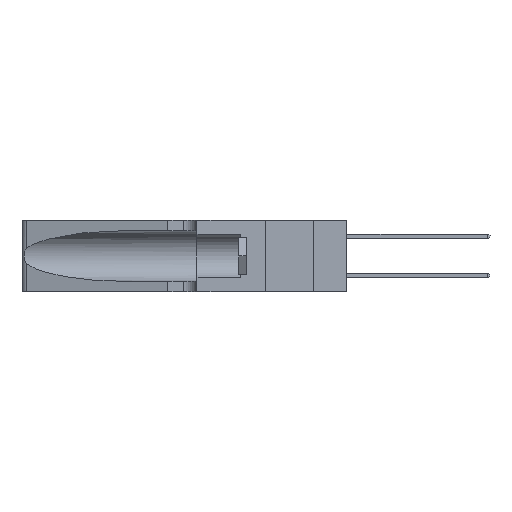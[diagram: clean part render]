
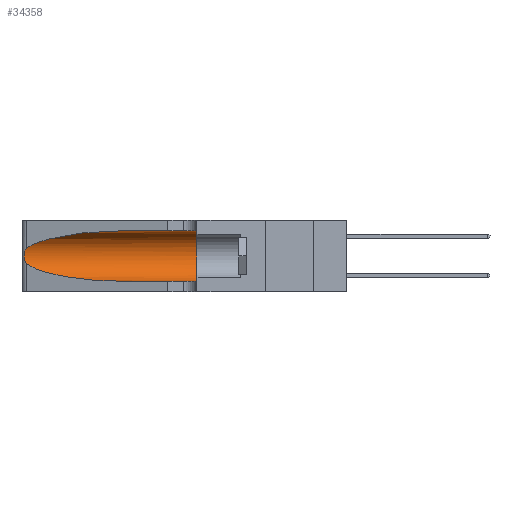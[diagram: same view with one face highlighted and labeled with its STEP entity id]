
A CAD part, left-side view. The second image highlights one B-rep face of the part: STEP entity #34358.
In plain terms, the highlighted cylindrical face has radius 3.308 mm (diameter 6.617 mm), a partial arc.
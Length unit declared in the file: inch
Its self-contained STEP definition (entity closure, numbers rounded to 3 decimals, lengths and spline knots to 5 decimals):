
#531 = ORIENTED_EDGE ( 'NONE', *, *, #25569, .T. ) ;
#635 = DIRECTION ( 'NONE',  ( 0., -1., 0. ) ) ;
#1025 = EDGE_CURVE ( 'NONE', #2782, #19241, #13619, .T. ) ;
#1356 = CARTESIAN_POINT ( 'NONE',  ( 0.1305, 0.35, 0.31525 ) ) ;
#1632 = CARTESIAN_POINT ( 'NONE',  ( 0.1305, 0.72297, 0.05475 ) ) ;
#2381 = CARTESIAN_POINT ( 'NONE',  ( 0.25487, 1.22718, 0.14631 ) ) ;
#2574 = AXIS2_PLACEMENT_3D ( 'NONE', #5266, #4666, #28445 ) ;
#2782 = VERTEX_POINT ( 'NONE', #18855 ) ;
#3569 = VERTEX_POINT ( 'NONE', #1356 ) ;
#4320 = CARTESIAN_POINT ( 'NONE',  ( 0.2373, 1.15595, 0.28018 ) ) ;
#4666 = DIRECTION ( 'NONE',  ( 0., 1., 0. ) ) ;
#5266 = CARTESIAN_POINT ( 'NONE',  ( 0.1305, 0.35, 0.185 ) ) ;
#6025 = CARTESIAN_POINT ( 'NONE',  ( 0.26017, 1.23833, 0.17102 ) ) ;
#6101 = ORIENTED_EDGE ( 'NONE', *, *, #24905, .T. ) ;
#6287 = ORIENTED_EDGE ( 'NONE', *, *, #32397, .F. ) ;
#6356 = VERTEX_POINT ( 'NONE', #2381 ) ;
#6449 = CARTESIAN_POINT ( 'NONE',  ( 0.25639, 1.23186, 0.15144 ) ) ;
#8166 = CARTESIAN_POINT ( 'NONE',  ( 0.1305, 0.72297, 0.31525 ) ) ;
#9564 = CARTESIAN_POINT ( 'NONE',  ( 0.25856, 1.23593, 0.16098 ) ) ;
#9710 = CARTESIAN_POINT ( 'NONE',  ( 0.26075, 1.23896, 0.19203 ) ) ;
#11572 = CIRCLE ( 'NONE', #2574, 0.13025 ) ;
#12042 = CARTESIAN_POINT ( 'NONE',  ( 0.25487, 1.22718, 0.14631 ) ) ;
#13156 = VERTEX_POINT ( 'NONE', #18201 ) ;
#13256 = CARTESIAN_POINT ( 'NONE',  ( 0.25487, 1.22718, 0.14631 ) ) ;
#13619 =( BOUNDED_CURVE ( )  B_SPLINE_CURVE ( 3, ( #8166, #24989, #4320, #18243 ),
 .UNSPECIFIED., .F., .F. ) 
 B_SPLINE_CURVE_WITH_KNOTS ( ( 4, 4 ),
 ( 1.5708, 2.84003 ),
 .UNSPECIFIED. ) 
 CURVE ( )  GEOMETRIC_REPRESENTATION_ITEM ( )  RATIONAL_B_SPLINE_CURVE ( ( 1., 0.87, 0.87, 1. ) ) 
 REPRESENTATION_ITEM ( '' )  );
#13638 = VECTOR ( 'NONE', #31619, 39.37008 ) ;
#15139 = CARTESIAN_POINT ( 'NONE',  ( 0.25639, 1.23184, 0.21858 ) ) ;
#15176 = CYLINDRICAL_SURFACE ( 'NONE', #16251, 0.13025 ) ;
#15279 = CARTESIAN_POINT ( 'NONE',  ( 0.25787, 1.23484, 0.2124 ) ) ;
#15413 = EDGE_CURVE ( 'NONE', #2782, #3569, #27504, .T. ) ;
#15910 = DIRECTION ( 'NONE',  ( 0., 0., -1. ) ) ;
#16251 = AXIS2_PLACEMENT_3D ( 'NONE', #25642, #19061, #15910 ) ;
#18201 = CARTESIAN_POINT ( 'NONE',  ( 0.1305, 0.35, 0.05475 ) ) ;
#18243 = CARTESIAN_POINT ( 'NONE',  ( 0.25487, 1.22718, 0.22369 ) ) ;
#18705 = CARTESIAN_POINT ( 'NONE',  ( 0.25854, 1.2359, 0.20912 ) ) ;
#18855 = CARTESIAN_POINT ( 'NONE',  ( 0.1305, 0.72297, 0.31525 ) ) ;
#19061 = DIRECTION ( 'NONE',  ( 0., -1., 0. ) ) ;
#19241 = VERTEX_POINT ( 'NONE', #28084 ) ;
#20495 = FACE_OUTER_BOUND ( 'NONE', #32352, .T. ) ;
#22337 = CARTESIAN_POINT ( 'NONE',  ( 0.2373, 1.15595, 0.08982 ) ) ;
#24264 = B_SPLINE_CURVE_WITH_KNOTS ( 'NONE', 3,
 ( #28708, #35617, #15139, #15279, #18705, #30000, #9710, #26829, #6025, #9564, #40023, #6449, #33584, #13256 ),
 .UNSPECIFIED., .F., .F.,
 ( 4, 2, 2, 2, 2, 2, 4 ),
 ( 0., 0.00027, 0.00053, 0.00107, 0.0016, 0.00187, 0.00214 ),
 .UNSPECIFIED. ) ;
#24905 = EDGE_CURVE ( 'NONE', #19241, #6356, #24264, .T. ) ;
#24989 = CARTESIAN_POINT ( 'NONE',  ( 0.18966, 0.96281, 0.31525 ) ) ;
#25569 = EDGE_CURVE ( 'NONE', #6356, #31322, #42159, .T. ) ;
#25642 = CARTESIAN_POINT ( 'NONE',  ( 0.1305, 1.61858, 0.185 ) ) ;
#26042 = EDGE_CURVE ( 'NONE', #31322, #13156, #37537, .T. ) ;
#26687 = ORIENTED_EDGE ( 'NONE', *, *, #15413, .F. ) ;
#26829 = CARTESIAN_POINT ( 'NONE',  ( 0.26075, 1.23896, 0.178 ) ) ;
#27504 = LINE ( 'NONE', #41184, #13638 ) ;
#27622 = ORIENTED_EDGE ( 'NONE', *, *, #26042, .T. ) ;
#28084 = CARTESIAN_POINT ( 'NONE',  ( 0.25487, 1.22718, 0.22369 ) ) ;
#28445 = DIRECTION ( 'NONE',  ( 0., 0., 1. ) ) ;
#28708 = CARTESIAN_POINT ( 'NONE',  ( 0.25487, 1.22718, 0.22369 ) ) ;
#30000 = CARTESIAN_POINT ( 'NONE',  ( 0.26018, 1.23835, 0.19895 ) ) ;
#31130 = VECTOR ( 'NONE', #635, 39.37008 ) ;
#31322 = VERTEX_POINT ( 'NONE', #34382 ) ;
#31461 = CARTESIAN_POINT ( 'NONE',  ( 0.1305, 1.61858, 0.05475 ) ) ;
#31619 = DIRECTION ( 'NONE',  ( 0., -1., 0. ) ) ;
#32352 = EDGE_LOOP ( 'NONE', ( #43998, #6101, #531, #27622, #6287, #26687 ) ) ;
#32397 = EDGE_CURVE ( 'NONE', #3569, #13156, #11572, .T. ) ;
#33584 = CARTESIAN_POINT ( 'NONE',  ( 0.25555, 1.22993, 0.14849 ) ) ;
#34358 = ADVANCED_FACE ( 'NONE', ( #20495 ), #15176, .F. ) ;
#34382 = CARTESIAN_POINT ( 'NONE',  ( 0.1305, 0.72297, 0.05475 ) ) ;
#35617 = CARTESIAN_POINT ( 'NONE',  ( 0.25555, 1.22994, 0.2215 ) ) ;
#37537 = LINE ( 'NONE', #31461, #31130 ) ;
#40023 = CARTESIAN_POINT ( 'NONE',  ( 0.25789, 1.23486, 0.15765 ) ) ;
#41184 = CARTESIAN_POINT ( 'NONE',  ( 0.1305, 1.61858, 0.31525 ) ) ;
#42159 =( BOUNDED_CURVE ( )  B_SPLINE_CURVE ( 3, ( #12042, #22337, #42706, #1632 ),
 .UNSPECIFIED., .F., .T. ) 
 B_SPLINE_CURVE_WITH_KNOTS ( ( 4, 4 ),
 ( 3.44316, 4.71239 ),
 .UNSPECIFIED. ) 
 CURVE ( )  GEOMETRIC_REPRESENTATION_ITEM ( )  RATIONAL_B_SPLINE_CURVE ( ( 1., 0.87, 0.87, 1. ) ) 
 REPRESENTATION_ITEM ( '' )  );
#42706 = CARTESIAN_POINT ( 'NONE',  ( 0.18966, 0.96281, 0.05475 ) ) ;
#43998 = ORIENTED_EDGE ( 'NONE', *, *, #1025, .T. ) ;
